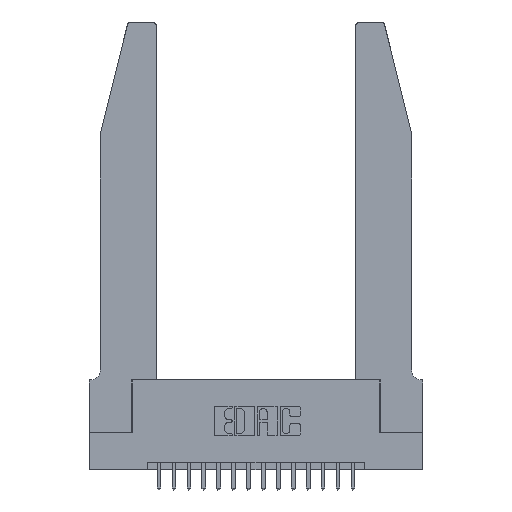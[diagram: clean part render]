
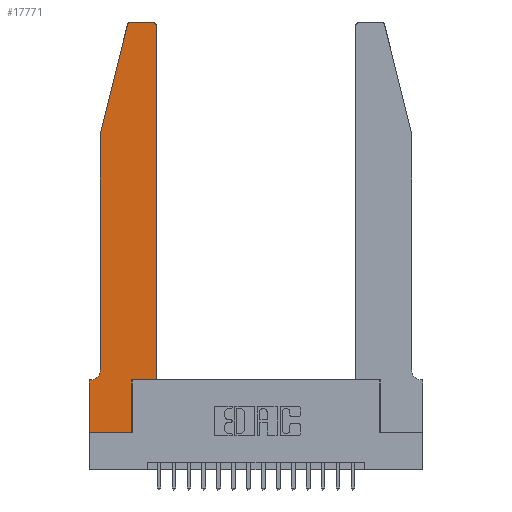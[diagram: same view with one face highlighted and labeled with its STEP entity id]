
A CAD part, top view. The second image highlights one B-rep face of the part: STEP entity #17771.
In plain terms, the highlighted planar face has unit normal (0, 0, 1).
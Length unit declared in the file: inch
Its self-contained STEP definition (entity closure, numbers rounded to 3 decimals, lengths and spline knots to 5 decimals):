
#34 = ORIENTED_EDGE ( 'NONE', *, *, #4289, .T. ) ;
#115 = PLANE ( 'NONE',  #798 ) ;
#314 = EDGE_CURVE ( 'NONE', #18752, #18634, #7324, .T. ) ;
#403 = LINE ( 'NONE', #5993, #12594 ) ;
#798 = AXIS2_PLACEMENT_3D ( 'NONE', #15265, #1699, #12364 ) ;
#1204 = DIRECTION ( 'NONE',  ( 0., 1., 0. ) ) ;
#1532 = CARTESIAN_POINT ( 'NONE',  ( 0.2605, 2.75, 0.37 ) ) ;
#1585 = VECTOR ( 'NONE', #18084, 39.37008 ) ;
#1622 = EDGE_CURVE ( 'NONE', #14369, #13047, #14382, .T. ) ;
#1699 = DIRECTION ( 'NONE',  ( 0., 0., 1. ) ) ;
#1753 = ORIENTED_EDGE ( 'NONE', *, *, #314, .T. ) ;
#2411 = CARTESIAN_POINT ( 'NONE',  ( 0.4205, 2.75, 0.37 ) ) ;
#2619 = EDGE_CURVE ( 'NONE', #6258, #3383, #14341, .T. ) ;
#2722 = ORIENTED_EDGE ( 'NONE', *, *, #4788, .T. ) ;
#3264 = DIRECTION ( 'NONE',  ( 0., -1., 0. ) ) ;
#3383 = VERTEX_POINT ( 'NONE', #10134 ) ;
#4022 = AXIS2_PLACEMENT_3D ( 'NONE', #17926, #8982, #19369 ) ;
#4289 = EDGE_CURVE ( 'NONE', #3383, #17747, #10989, .T. ) ;
#4744 = VERTEX_POINT ( 'NONE', #16317 ) ;
#4788 = EDGE_CURVE ( 'NONE', #11292, #6258, #17507, .T. ) ;
#4915 = EDGE_LOOP ( 'NONE', ( #12009, #17372, #1753, #14346, #2722, #15729, #34, #12726, #16698, #6099, #6556, #11544 ) ) ;
#5306 = DIRECTION ( 'NONE',  ( -0.239, -0.971, 0. ) ) ;
#5576 = CARTESIAN_POINT ( 'NONE',  ( 0.4205, 2.72, 0.37 ) ) ;
#5648 = VERTEX_POINT ( 'NONE', #18206 ) ;
#5661 = AXIS2_PLACEMENT_3D ( 'NONE', #8971, #19359, #10489 ) ;
#5834 = CARTESIAN_POINT ( 'NONE',  ( 0.0055, 0.35, 0.37 ) ) ;
#5993 = CARTESIAN_POINT ( 'NONE',  ( 0.0755, 2., 0.37 ) ) ;
#6071 = CARTESIAN_POINT ( 'NONE',  ( 0.0755, 2., 0.37 ) ) ;
#6099 = ORIENTED_EDGE ( 'NONE', *, *, #1622, .T. ) ;
#6258 = VERTEX_POINT ( 'NONE', #5834 ) ;
#6556 = ORIENTED_EDGE ( 'NONE', *, *, #17542, .T. ) ;
#7068 = DIRECTION ( 'NONE',  ( 1., 0., 0. ) ) ;
#7324 = LINE ( 'NONE', #6071, #14869 ) ;
#7437 = VECTOR ( 'NONE', #3264, 39.37008 ) ;
#7504 = EDGE_CURVE ( 'NONE', #5648, #14369, #12085, .T. ) ;
#7797 = VERTEX_POINT ( 'NONE', #16950 ) ;
#7831 = CARTESIAN_POINT ( 'NONE',  ( 0., 0., 0.37 ) ) ;
#8084 = DIRECTION ( 'NONE',  ( -1., 0., 0. ) ) ;
#8326 = CARTESIAN_POINT ( 'NONE',  ( 0.0755, 0.35, 0.37 ) ) ;
#8482 = CARTESIAN_POINT ( 'NONE',  ( 0.2865, 0.35, 0.37 ) ) ;
#8643 = CARTESIAN_POINT ( 'NONE',  ( 0.4505, 0.35, 0.37 ) ) ;
#8915 = EDGE_CURVE ( 'NONE', #18634, #11292, #403, .T. ) ;
#8971 = CARTESIAN_POINT ( 'NONE',  ( 0.0055, 0.42, 0.37 ) ) ;
#8982 = DIRECTION ( 'NONE',  ( 0., 0., 1. ) ) ;
#9241 = CARTESIAN_POINT ( 'NONE',  ( 0., 0., 0.37 ) ) ;
#9926 = VERTEX_POINT ( 'NONE', #2411 ) ;
#10074 = EDGE_CURVE ( 'NONE', #17747, #5648, #14171, .T. ) ;
#10100 = EDGE_CURVE ( 'NONE', #9926, #4744, #17208, .T. ) ;
#10134 = CARTESIAN_POINT ( 'NONE',  ( 0., 0.35, 0.37 ) ) ;
#10172 = DIRECTION ( 'NONE',  ( 0., 1., 0. ) ) ;
#10248 = AXIS2_PLACEMENT_3D ( 'NONE', #5576, #16092, #7068 ) ;
#10346 = CARTESIAN_POINT ( 'NONE',  ( 0.0755, 2., 0.37 ) ) ;
#10388 = VECTOR ( 'NONE', #18195, 39.37008 ) ;
#10489 = DIRECTION ( 'NONE',  ( -1., 0., 0. ) ) ;
#10989 = LINE ( 'NONE', #7831, #7437 ) ;
#11292 = VERTEX_POINT ( 'NONE', #12420 ) ;
#11544 = ORIENTED_EDGE ( 'NONE', *, *, #16155, .T. ) ;
#11798 = LINE ( 'NONE', #8643, #19197 ) ;
#12009 = ORIENTED_EDGE ( 'NONE', *, *, #10100, .T. ) ;
#12085 = LINE ( 'NONE', #19164, #19447 ) ;
#12122 = CARTESIAN_POINT ( 'NONE',  ( 0.25487, 2.72718, 0.37 ) ) ;
#12364 = DIRECTION ( 'NONE',  ( 1., 0., 0. ) ) ;
#12420 = CARTESIAN_POINT ( 'NONE',  ( 0.0755, 0.42, 0.37 ) ) ;
#12517 = FACE_OUTER_BOUND ( 'NONE', #4915, .T. ) ;
#12594 = VECTOR ( 'NONE', #16518, 39.37008 ) ;
#12726 = ORIENTED_EDGE ( 'NONE', *, *, #10074, .T. ) ;
#13047 = VERTEX_POINT ( 'NONE', #15489 ) ;
#13619 = CARTESIAN_POINT ( 'NONE',  ( 0., 0., 0.37 ) ) ;
#13699 = VECTOR ( 'NONE', #15101, 39.37008 ) ;
#14164 = CIRCLE ( 'NONE', #4022, 0.03 ) ;
#14171 = LINE ( 'NONE', #13619, #13699 ) ;
#14341 = LINE ( 'NONE', #8326, #17368 ) ;
#14346 = ORIENTED_EDGE ( 'NONE', *, *, #8915, .T. ) ;
#14369 = VERTEX_POINT ( 'NONE', #8482 ) ;
#14382 = LINE ( 'NONE', #17786, #10388 ) ;
#14869 = VECTOR ( 'NONE', #5306, 39.37008 ) ;
#14881 = CIRCLE ( 'NONE', #10248, 0.03 ) ;
#15101 = DIRECTION ( 'NONE',  ( 1., 0., 0. ) ) ;
#15265 = CARTESIAN_POINT ( 'NONE',  ( 0., 0.35, 0.37 ) ) ;
#15489 = CARTESIAN_POINT ( 'NONE',  ( 0.4505, 0.35, 0.37 ) ) ;
#15729 = ORIENTED_EDGE ( 'NONE', *, *, #2619, .T. ) ;
#16092 = DIRECTION ( 'NONE',  ( 0., 0., 1. ) ) ;
#16155 = EDGE_CURVE ( 'NONE', #7797, #9926, #14881, .T. ) ;
#16317 = CARTESIAN_POINT ( 'NONE',  ( 0.284, 2.75, 0.37 ) ) ;
#16518 = DIRECTION ( 'NONE',  ( 0., -1., 0. ) ) ;
#16698 = ORIENTED_EDGE ( 'NONE', *, *, #7504, .T. ) ;
#16908 = EDGE_CURVE ( 'NONE', #4744, #18752, #14164, .T. ) ;
#16950 = CARTESIAN_POINT ( 'NONE',  ( 0.4505, 2.72, 0.37 ) ) ;
#17208 = LINE ( 'NONE', #1532, #1585 ) ;
#17368 = VECTOR ( 'NONE', #8084, 39.37008 ) ;
#17372 = ORIENTED_EDGE ( 'NONE', *, *, #16908, .T. ) ;
#17507 = CIRCLE ( 'NONE', #5661, 0.07 ) ;
#17542 = EDGE_CURVE ( 'NONE', #13047, #7797, #11798, .T. ) ;
#17747 = VERTEX_POINT ( 'NONE', #9241 ) ;
#17771 = ADVANCED_FACE ( 'NONE', ( #12517 ), #115, .T. ) ;
#17786 = CARTESIAN_POINT ( 'NONE',  ( 0.4505, 0.35, 0.37 ) ) ;
#17926 = CARTESIAN_POINT ( 'NONE',  ( 0.284, 2.72, 0.37 ) ) ;
#18084 = DIRECTION ( 'NONE',  ( -1., 0., 0. ) ) ;
#18195 = DIRECTION ( 'NONE',  ( 1., 0., 0. ) ) ;
#18206 = CARTESIAN_POINT ( 'NONE',  ( 0.2865, 0., 0.37 ) ) ;
#18634 = VERTEX_POINT ( 'NONE', #10346 ) ;
#18752 = VERTEX_POINT ( 'NONE', #12122 ) ;
#19164 = CARTESIAN_POINT ( 'NONE',  ( 0.2865, 0.35, 0.37 ) ) ;
#19197 = VECTOR ( 'NONE', #10172, 39.37008 ) ;
#19359 = DIRECTION ( 'NONE',  ( 0., 0., -1. ) ) ;
#19369 = DIRECTION ( 'NONE',  ( 1., 0., 0. ) ) ;
#19447 = VECTOR ( 'NONE', #1204, 39.37008 ) ;
